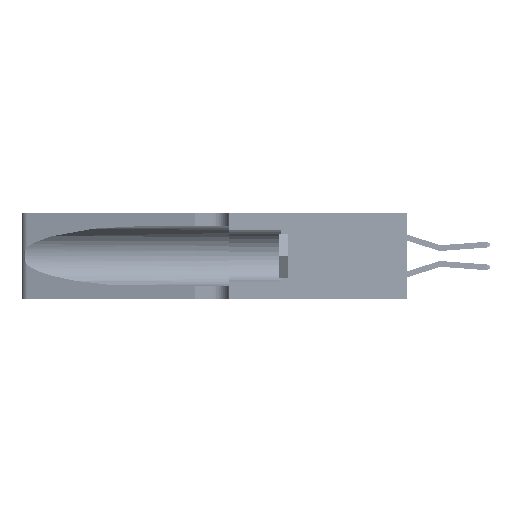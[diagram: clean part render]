
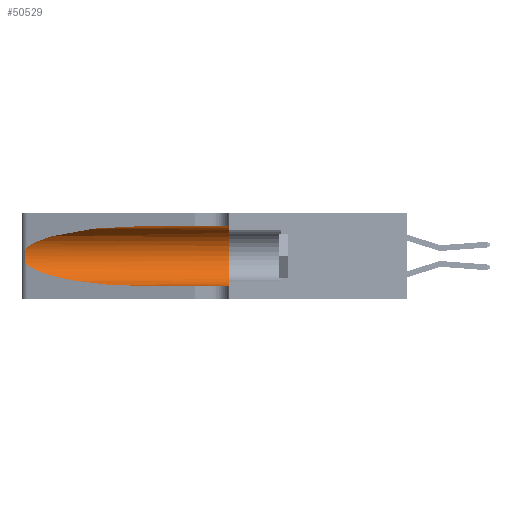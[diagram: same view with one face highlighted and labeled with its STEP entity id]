
A CAD part, left-side view. The second image highlights one B-rep face of the part: STEP entity #50529.
In plain terms, the highlighted cylindrical face has radius 3.308 mm (diameter 6.617 mm), a partial arc.
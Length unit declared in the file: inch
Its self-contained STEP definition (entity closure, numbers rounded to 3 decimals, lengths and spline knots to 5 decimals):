
#194 = ORIENTED_EDGE ( 'NONE', *, *, #21342, .T. ) ;
#2036 = LINE ( 'NONE', #48204, #15126 ) ;
#2711 = VERTEX_POINT ( 'NONE', #35369 ) ;
#2973 = VECTOR ( 'NONE', #4410, 39.37008 ) ;
#4410 = DIRECTION ( 'NONE',  ( 0., -1., 0. ) ) ;
#4429 = CARTESIAN_POINT ( 'NONE',  ( 0.2373, 1.15595, 0.28018 ) ) ;
#4803 = ORIENTED_EDGE ( 'NONE', *, *, #23128, .T. ) ;
#5595 = ORIENTED_EDGE ( 'NONE', *, *, #26567, .F. ) ;
#6493 = DIRECTION ( 'NONE',  ( 0., 1., 0. ) ) ;
#6958 = CARTESIAN_POINT ( 'NONE',  ( 0.1305, 0.72297, 0.05475 ) ) ;
#7345 = VERTEX_POINT ( 'NONE', #42305 ) ;
#7465 = CARTESIAN_POINT ( 'NONE',  ( 0.2373, 1.15595, 0.08982 ) ) ;
#8612 = DIRECTION ( 'NONE',  ( 0., -1., 0. ) ) ;
#9270 = AXIS2_PLACEMENT_3D ( 'NONE', #10328, #6493, #18677 ) ;
#9639 = EDGE_CURVE ( 'NONE', #7345, #34618, #15601, .T. ) ;
#10328 = CARTESIAN_POINT ( 'NONE',  ( 0.1305, 0.35, 0.185 ) ) ;
#10769 = CARTESIAN_POINT ( 'NONE',  ( 0.25639, 1.23184, 0.21858 ) ) ;
#11630 = CARTESIAN_POINT ( 'NONE',  ( 0.25487, 1.22718, 0.14631 ) ) ;
#15126 = VECTOR ( 'NONE', #8612, 39.37008 ) ;
#15316 = CARTESIAN_POINT ( 'NONE',  ( 0.26017, 1.23833, 0.17102 ) ) ;
#15601 =( BOUNDED_CURVE ( )  B_SPLINE_CURVE ( 3, ( #48856, #39486, #4429, #36300 ),
 .UNSPECIFIED., .F., .T. ) 
 B_SPLINE_CURVE_WITH_KNOTS ( ( 4, 4 ),
 ( 1.5708, 2.84003 ),
 .UNSPECIFIED. ) 
 CURVE ( )  GEOMETRIC_REPRESENTATION_ITEM ( )  RATIONAL_B_SPLINE_CURVE ( ( 1., 0.87, 0.87, 1. ) ) 
 REPRESENTATION_ITEM ( '' )  );
#18278 = CARTESIAN_POINT ( 'NONE',  ( 0.26018, 1.23835, 0.19895 ) ) ;
#18677 = DIRECTION ( 'NONE',  ( 0., 0., 1. ) ) ;
#18798 = CARTESIAN_POINT ( 'NONE',  ( 0.25854, 1.2359, 0.20912 ) ) ;
#19142 = CARTESIAN_POINT ( 'NONE',  ( 0.25487, 1.22718, 0.14631 ) ) ;
#20183 = CARTESIAN_POINT ( 'NONE',  ( 0.25487, 1.22718, 0.22369 ) ) ;
#20623 = AXIS2_PLACEMENT_3D ( 'NONE', #32027, #24168, #44069 ) ;
#21342 = EDGE_CURVE ( 'NONE', #48498, #27525, #31875, .T. ) ;
#21668 = ORIENTED_EDGE ( 'NONE', *, *, #9639, .T. ) ;
#22788 = CARTESIAN_POINT ( 'NONE',  ( 0.26075, 1.23896, 0.178 ) ) ;
#23128 = EDGE_CURVE ( 'NONE', #27525, #24826, #28499, .T. ) ;
#23480 = CARTESIAN_POINT ( 'NONE',  ( 0.25856, 1.23593, 0.16098 ) ) ;
#24168 = DIRECTION ( 'NONE',  ( 0., -1., 0. ) ) ;
#24571 = EDGE_LOOP ( 'NONE', ( #21668, #30669, #194, #4803, #5595, #30564 ) ) ;
#24826 = VERTEX_POINT ( 'NONE', #30917 ) ;
#26567 = EDGE_CURVE ( 'NONE', #2711, #24826, #50023, .T. ) ;
#27143 = CARTESIAN_POINT ( 'NONE',  ( 0.25555, 1.22993, 0.14849 ) ) ;
#27525 = VERTEX_POINT ( 'NONE', #39914 ) ;
#27655 = CARTESIAN_POINT ( 'NONE',  ( 0.25639, 1.23186, 0.15144 ) ) ;
#28499 = LINE ( 'NONE', #40345, #2973 ) ;
#30564 = ORIENTED_EDGE ( 'NONE', *, *, #35808, .F. ) ;
#30669 = ORIENTED_EDGE ( 'NONE', *, *, #38751, .T. ) ;
#30917 = CARTESIAN_POINT ( 'NONE',  ( 0.1305, 0.35, 0.05475 ) ) ;
#31875 =( BOUNDED_CURVE ( )  B_SPLINE_CURVE ( 3, ( #19142, #7465, #39412, #6958 ),
 .UNSPECIFIED., .F., .F. ) 
 B_SPLINE_CURVE_WITH_KNOTS ( ( 4, 4 ),
 ( 3.44316, 4.71239 ),
 .UNSPECIFIED. ) 
 CURVE ( )  GEOMETRIC_REPRESENTATION_ITEM ( )  RATIONAL_B_SPLINE_CURVE ( ( 1., 0.87, 0.87, 1. ) ) 
 REPRESENTATION_ITEM ( '' )  );
#32027 = CARTESIAN_POINT ( 'NONE',  ( 0.1305, 1.61858, 0.185 ) ) ;
#32357 = FACE_OUTER_BOUND ( 'NONE', #24571, .T. ) ;
#34618 = VERTEX_POINT ( 'NONE', #20183 ) ;
#34854 = CYLINDRICAL_SURFACE ( 'NONE', #20623, 0.13025 ) ;
#35369 = CARTESIAN_POINT ( 'NONE',  ( 0.1305, 0.35, 0.31525 ) ) ;
#35689 = CARTESIAN_POINT ( 'NONE',  ( 0.25487, 1.22718, 0.14631 ) ) ;
#35808 = EDGE_CURVE ( 'NONE', #7345, #2711, #2036, .T. ) ;
#36300 = CARTESIAN_POINT ( 'NONE',  ( 0.25487, 1.22718, 0.22369 ) ) ;
#38751 = EDGE_CURVE ( 'NONE', #34618, #48498, #47251, .T. ) ;
#39412 = CARTESIAN_POINT ( 'NONE',  ( 0.18966, 0.96281, 0.05475 ) ) ;
#39486 = CARTESIAN_POINT ( 'NONE',  ( 0.18966, 0.96281, 0.31525 ) ) ;
#39914 = CARTESIAN_POINT ( 'NONE',  ( 0.1305, 0.72297, 0.05475 ) ) ;
#40345 = CARTESIAN_POINT ( 'NONE',  ( 0.1305, 1.61858, 0.05475 ) ) ;
#42305 = CARTESIAN_POINT ( 'NONE',  ( 0.1305, 0.72297, 0.31525 ) ) ;
#42722 = CARTESIAN_POINT ( 'NONE',  ( 0.25787, 1.23484, 0.2124 ) ) ;
#43383 = CARTESIAN_POINT ( 'NONE',  ( 0.25789, 1.23486, 0.15765 ) ) ;
#44069 = DIRECTION ( 'NONE',  ( 0., 0., -1. ) ) ;
#46532 = CARTESIAN_POINT ( 'NONE',  ( 0.25555, 1.22994, 0.2215 ) ) ;
#46707 = CARTESIAN_POINT ( 'NONE',  ( 0.26075, 1.23896, 0.19203 ) ) ;
#47251 = B_SPLINE_CURVE_WITH_KNOTS ( 'NONE', 3,
 ( #50403, #46532, #10769, #42722, #18798, #18278, #46707, #22788, #15316, #23480, #43383, #27655, #27143, #11630 ),
 .UNSPECIFIED., .F., .F.,
 ( 4, 2, 2, 2, 2, 2, 4 ),
 ( 0., 0.00027, 0.00053, 0.00107, 0.0016, 0.00187, 0.00214 ),
 .UNSPECIFIED. ) ;
#48204 = CARTESIAN_POINT ( 'NONE',  ( 0.1305, 1.61858, 0.31525 ) ) ;
#48498 = VERTEX_POINT ( 'NONE', #35689 ) ;
#48856 = CARTESIAN_POINT ( 'NONE',  ( 0.1305, 0.72297, 0.31525 ) ) ;
#50023 = CIRCLE ( 'NONE', #9270, 0.13025 ) ;
#50403 = CARTESIAN_POINT ( 'NONE',  ( 0.25487, 1.22718, 0.22369 ) ) ;
#50529 = ADVANCED_FACE ( 'NONE', ( #32357 ), #34854, .F. ) ;
